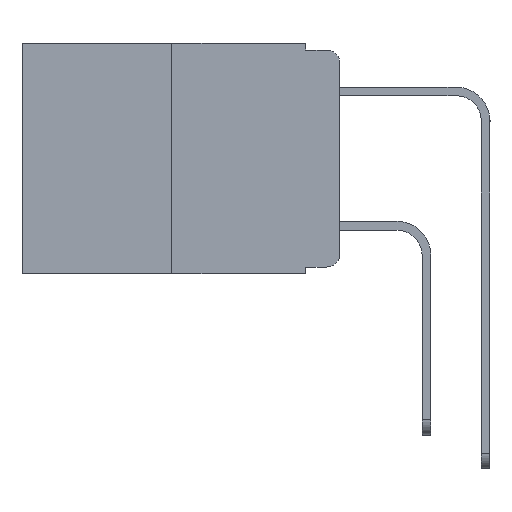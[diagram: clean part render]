
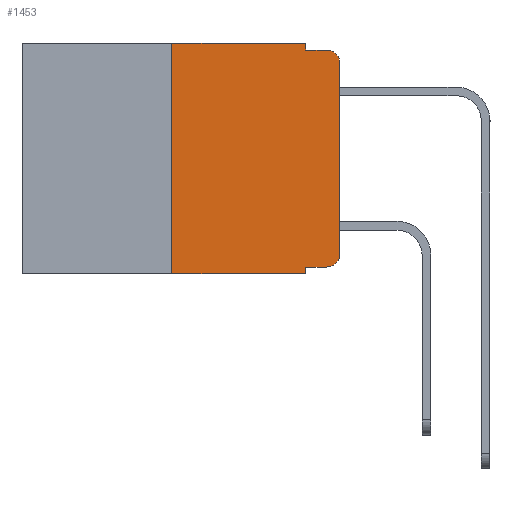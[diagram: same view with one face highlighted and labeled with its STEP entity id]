
A CAD part, left-side view. The second image highlights one B-rep face of the part: STEP entity #1453.
In plain terms, the highlighted planar face has unit normal (-1, 0, 0).
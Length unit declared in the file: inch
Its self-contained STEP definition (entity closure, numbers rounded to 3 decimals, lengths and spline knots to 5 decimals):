
#658 = VERTEX_POINT ( 'NONE', #20383 ) ;
#1410 = PLANE ( 'NONE',  #14253 ) ;
#1453 = ADVANCED_FACE ( 'NONE', ( #3013 ), #1410, .F. ) ;
#1924 = VECTOR ( 'NONE', #19686, 39.37008 ) ;
#2129 = EDGE_CURVE ( 'NONE', #23166, #14291, #22584, .T. ) ;
#2459 = CARTESIAN_POINT ( 'NONE',  ( 0., 0.051, -0.333 ) ) ;
#2549 = EDGE_CURVE ( 'NONE', #658, #14011, #21111, .T. ) ;
#2701 = CARTESIAN_POINT ( 'NONE',  ( 0., 0.02, -0.01 ) ) ;
#2807 = VECTOR ( 'NONE', #18475, 39.37008 ) ;
#2846 = VERTEX_POINT ( 'NONE', #20277 ) ;
#2992 = EDGE_LOOP ( 'NONE', ( #16703, #4804, #17017, #4506, #17316, #9864, #16435, #3918, #21162, #5147 ) ) ;
#3013 = FACE_OUTER_BOUND ( 'NONE', #2992, .T. ) ;
#3401 = DIRECTION ( 'NONE',  ( 0., -1., 0. ) ) ;
#3918 = ORIENTED_EDGE ( 'NONE', *, *, #5281, .F. ) ;
#4506 = ORIENTED_EDGE ( 'NONE', *, *, #5090, .F. ) ;
#4804 = ORIENTED_EDGE ( 'NONE', *, *, #8754, .T. ) ;
#4974 = AXIS2_PLACEMENT_3D ( 'NONE', #6783, #19751, #8702 ) ;
#5090 = EDGE_CURVE ( 'NONE', #2846, #17008, #19491, .T. ) ;
#5147 = ORIENTED_EDGE ( 'NONE', *, *, #22155, .T. ) ;
#5281 = EDGE_CURVE ( 'NONE', #658, #14291, #14320, .T. ) ;
#5292 = DIRECTION ( 'NONE',  ( 1., 0., 0. ) ) ;
#6178 = CARTESIAN_POINT ( 'NONE',  ( 0., 0.25, 0. ) ) ;
#6716 = CARTESIAN_POINT ( 'NONE',  ( 0., 0.473, 0. ) ) ;
#6783 = CARTESIAN_POINT ( 'NONE',  ( 0., 0.02, -0.313 ) ) ;
#7790 = VECTOR ( 'NONE', #3401, 39.37008 ) ;
#7923 = LINE ( 'NONE', #11137, #2807 ) ;
#8271 = LINE ( 'NONE', #8600, #18074 ) ;
#8600 = CARTESIAN_POINT ( 'NONE',  ( 0., 0., 0. ) ) ;
#8620 = EDGE_CURVE ( 'NONE', #17008, #10178, #7923, .T. ) ;
#8702 = DIRECTION ( 'NONE',  ( 0., 0., -1. ) ) ;
#8754 = EDGE_CURVE ( 'NONE', #17059, #10178, #14768, .T. ) ;
#8788 = EDGE_CURVE ( 'NONE', #23166, #11449, #13630, .T. ) ;
#9383 = VECTOR ( 'NONE', #13486, 39.37008 ) ;
#9593 = CARTESIAN_POINT ( 'NONE',  ( 0., 0.051, -0.01 ) ) ;
#9776 = DIRECTION ( 'NONE',  ( -1., 0., 0. ) ) ;
#9864 = ORIENTED_EDGE ( 'NONE', *, *, #8788, .F. ) ;
#10178 = VERTEX_POINT ( 'NONE', #2701 ) ;
#11061 = CARTESIAN_POINT ( 'NONE',  ( 0., 0.051, 0. ) ) ;
#11137 = CARTESIAN_POINT ( 'NONE',  ( 0., 0.051, -0.01 ) ) ;
#11380 = CARTESIAN_POINT ( 'NONE',  ( 0., 0.25, -0.343 ) ) ;
#11449 = VERTEX_POINT ( 'NONE', #6178 ) ;
#11686 = DIRECTION ( 'NONE',  ( 0., 0., -1. ) ) ;
#11687 = CARTESIAN_POINT ( 'NONE',  ( 0., 0.25, 0. ) ) ;
#12499 = CARTESIAN_POINT ( 'NONE',  ( 0., 0.02, -0.333 ) ) ;
#13100 = CARTESIAN_POINT ( 'NONE',  ( 0., 0., -0.313 ) ) ;
#13411 = CARTESIAN_POINT ( 'NONE',  ( 0., 0.051, 0. ) ) ;
#13486 = DIRECTION ( 'NONE',  ( 0., 0., 1. ) ) ;
#13630 = LINE ( 'NONE', #11687, #9383 ) ;
#14011 = VERTEX_POINT ( 'NONE', #12499 ) ;
#14253 = AXIS2_PLACEMENT_3D ( 'NONE', #16396, #5292, #18289 ) ;
#14291 = VERTEX_POINT ( 'NONE', #18884 ) ;
#14320 = LINE ( 'NONE', #13411, #18143 ) ;
#14768 = CIRCLE ( 'NONE', #23914, 0.02 ) ;
#15490 = CIRCLE ( 'NONE', #4974, 0.02 ) ;
#15775 = EDGE_CURVE ( 'NONE', #19232, #17059, #8271, .T. ) ;
#16267 = LINE ( 'NONE', #6716, #1924 ) ;
#16396 = CARTESIAN_POINT ( 'NONE',  ( 0., 0.473, 0. ) ) ;
#16435 = ORIENTED_EDGE ( 'NONE', *, *, #2129, .T. ) ;
#16447 = CARTESIAN_POINT ( 'NONE',  ( 0., 0.473, -0.343 ) ) ;
#16703 = ORIENTED_EDGE ( 'NONE', *, *, #15775, .T. ) ;
#17008 = VERTEX_POINT ( 'NONE', #9593 ) ;
#17017 = ORIENTED_EDGE ( 'NONE', *, *, #8620, .F. ) ;
#17059 = VERTEX_POINT ( 'NONE', #18925 ) ;
#17316 = ORIENTED_EDGE ( 'NONE', *, *, #18546, .F. ) ;
#18074 = VECTOR ( 'NONE', #23404, 39.37008 ) ;
#18143 = VECTOR ( 'NONE', #11686, 39.37008 ) ;
#18289 = DIRECTION ( 'NONE',  ( 0., 0., -1. ) ) ;
#18474 = DIRECTION ( 'NONE',  ( 0., 0., -1. ) ) ;
#18475 = DIRECTION ( 'NONE',  ( 0., -1., 0. ) ) ;
#18546 = EDGE_CURVE ( 'NONE', #11449, #2846, #16267, .T. ) ;
#18884 = CARTESIAN_POINT ( 'NONE',  ( 0., 0.051, -0.343 ) ) ;
#18925 = CARTESIAN_POINT ( 'NONE',  ( 0., 0., -0.03 ) ) ;
#19232 = VERTEX_POINT ( 'NONE', #13100 ) ;
#19491 = LINE ( 'NONE', #11061, #22850 ) ;
#19686 = DIRECTION ( 'NONE',  ( 0., -1., 0. ) ) ;
#19751 = DIRECTION ( 'NONE',  ( -1., 0., 0. ) ) ;
#20277 = CARTESIAN_POINT ( 'NONE',  ( 0., 0.051, 0. ) ) ;
#20383 = CARTESIAN_POINT ( 'NONE',  ( 0., 0.051, -0.333 ) ) ;
#20845 = CARTESIAN_POINT ( 'NONE',  ( 0., 0.02, -0.03 ) ) ;
#21111 = LINE ( 'NONE', #2459, #24260 ) ;
#21162 = ORIENTED_EDGE ( 'NONE', *, *, #2549, .T. ) ;
#22155 = EDGE_CURVE ( 'NONE', #14011, #19232, #15490, .T. ) ;
#22584 = LINE ( 'NONE', #16447, #7790 ) ;
#22724 = DIRECTION ( 'NONE',  ( 0., 0., -1. ) ) ;
#22850 = VECTOR ( 'NONE', #18474, 39.37008 ) ;
#23081 = DIRECTION ( 'NONE',  ( 0., -1., 0. ) ) ;
#23166 = VERTEX_POINT ( 'NONE', #11380 ) ;
#23404 = DIRECTION ( 'NONE',  ( 0., 0., 1. ) ) ;
#23914 = AXIS2_PLACEMENT_3D ( 'NONE', #20845, #9776, #22724 ) ;
#24260 = VECTOR ( 'NONE', #23081, 39.37008 ) ;
